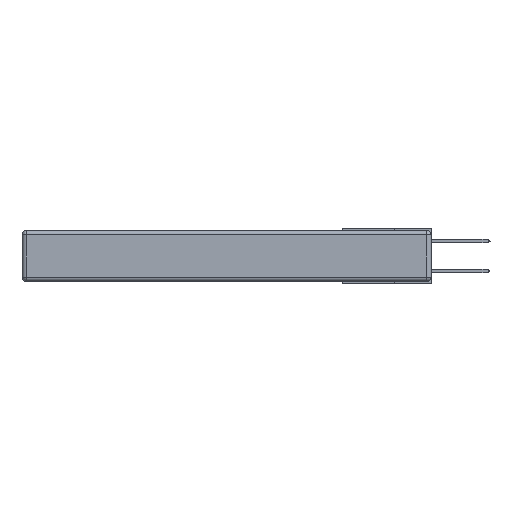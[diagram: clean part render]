
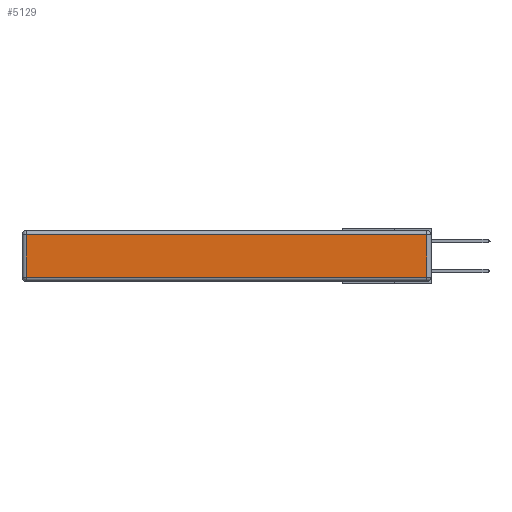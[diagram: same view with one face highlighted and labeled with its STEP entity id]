
A CAD part, left-side view. The second image highlights one B-rep face of the part: STEP entity #5129.
In plain terms, the highlighted planar face has unit normal (-1, 0, 0).
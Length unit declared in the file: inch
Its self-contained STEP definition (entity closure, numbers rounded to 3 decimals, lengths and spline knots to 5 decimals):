
#33 = CARTESIAN_POINT ( 'NONE',  ( 0., 2.75, -0.03 ) ) ;
#205 = CARTESIAN_POINT ( 'NONE',  ( 0., 0.03, -0.03 ) ) ;
#332 = CARTESIAN_POINT ( 'NONE',  ( 0., 2.72, -0.03 ) ) ;
#2408 = DIRECTION ( 'NONE',  ( 0., -1., 0. ) ) ;
#2521 = ORIENTED_EDGE ( 'NONE', *, *, #6486, .T. ) ;
#2747 = DIRECTION ( 'NONE',  ( 0., 1., 0. ) ) ;
#3923 = AXIS2_PLACEMENT_3D ( 'NONE', #4578, #9903, #14014 ) ;
#4304 = PLANE ( 'NONE',  #3923 ) ;
#4395 = CARTESIAN_POINT ( 'NONE',  ( 0., 2.72, -0.343 ) ) ;
#4578 = CARTESIAN_POINT ( 'NONE',  ( 0., 0., -0.343 ) ) ;
#4732 = VERTEX_POINT ( 'NONE', #332 ) ;
#4965 = LINE ( 'NONE', #33, #8692 ) ;
#4995 = VECTOR ( 'NONE', #2408, 39.37008 ) ;
#5129 = ADVANCED_FACE ( 'NONE', ( #12317 ), #4304, .T. ) ;
#5540 = ORIENTED_EDGE ( 'NONE', *, *, #7752, .T. ) ;
#6411 = EDGE_CURVE ( 'NONE', #7997, #4732, #4965, .T. ) ;
#6486 = EDGE_CURVE ( 'NONE', #8493, #7997, #16234, .T. ) ;
#6664 = CARTESIAN_POINT ( 'NONE',  ( 0., 2.72, -0.313 ) ) ;
#6942 = VECTOR ( 'NONE', #12697, 39.37008 ) ;
#7204 = DIRECTION ( 'NONE',  ( 0., 0., 1. ) ) ;
#7752 = EDGE_CURVE ( 'NONE', #4732, #14086, #8981, .T. ) ;
#7997 = VERTEX_POINT ( 'NONE', #205 ) ;
#8493 = VERTEX_POINT ( 'NONE', #10663 ) ;
#8692 = VECTOR ( 'NONE', #2747, 39.37008 ) ;
#8879 = ORIENTED_EDGE ( 'NONE', *, *, #14977, .T. ) ;
#8981 = LINE ( 'NONE', #4395, #6942 ) ;
#9903 = DIRECTION ( 'NONE',  ( -1., 0., 0. ) ) ;
#10611 = ORIENTED_EDGE ( 'NONE', *, *, #6411, .T. ) ;
#10663 = CARTESIAN_POINT ( 'NONE',  ( 0., 0.03, -0.313 ) ) ;
#12317 = FACE_OUTER_BOUND ( 'NONE', #13729, .T. ) ;
#12697 = DIRECTION ( 'NONE',  ( 0., 0., -1. ) ) ;
#13096 = VECTOR ( 'NONE', #7204, 39.37008 ) ;
#13729 = EDGE_LOOP ( 'NONE', ( #8879, #2521, #10611, #5540 ) ) ;
#14014 = DIRECTION ( 'NONE',  ( 0., 0., 1. ) ) ;
#14086 = VERTEX_POINT ( 'NONE', #6664 ) ;
#14977 = EDGE_CURVE ( 'NONE', #14086, #8493, #16035, .T. ) ;
#15057 = CARTESIAN_POINT ( 'NONE',  ( 0., 0.03, -0.343 ) ) ;
#15773 = CARTESIAN_POINT ( 'NONE',  ( 0., 0., -0.313 ) ) ;
#16035 = LINE ( 'NONE', #15773, #4995 ) ;
#16234 = LINE ( 'NONE', #15057, #13096 ) ;
